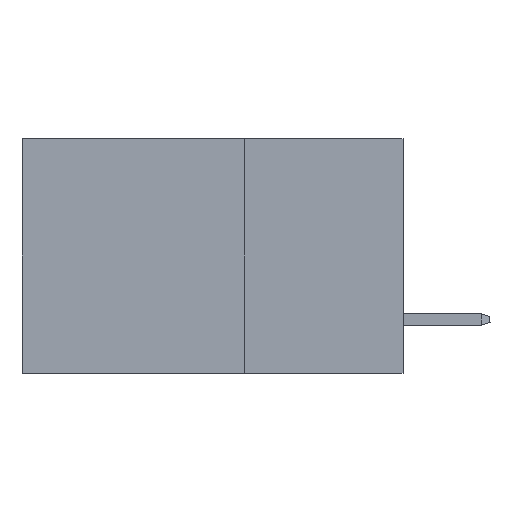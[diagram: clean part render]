
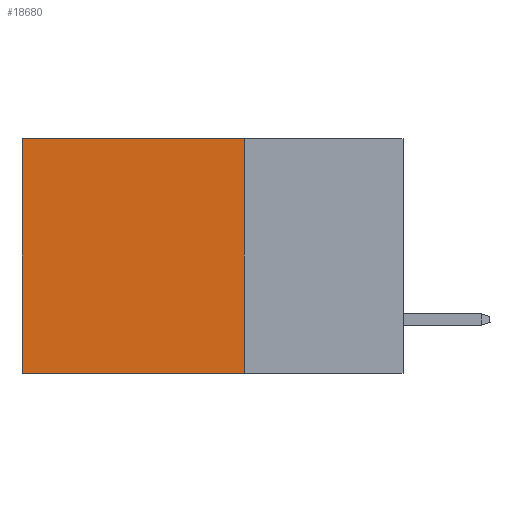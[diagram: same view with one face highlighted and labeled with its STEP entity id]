
A CAD part, left-side view. The second image highlights one B-rep face of the part: STEP entity #18680.
In plain terms, the highlighted planar face has unit normal (-1, 0, 0).
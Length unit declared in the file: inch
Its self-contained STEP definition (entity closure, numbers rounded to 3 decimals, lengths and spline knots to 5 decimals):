
#714 = VERTEX_POINT ( 'NONE', #31569 ) ;
#749 = EDGE_CURVE ( 'NONE', #714, #7709, #8805, .T. ) ;
#1723 = CARTESIAN_POINT ( 'NONE',  ( 0.2875, 0.25, -0.37 ) ) ;
#1878 = VECTOR ( 'NONE', #32065, 39.37008 ) ;
#2256 = EDGE_CURVE ( 'NONE', #714, #27507, #20958, .T. ) ;
#2496 = ORIENTED_EDGE ( 'NONE', *, *, #749, .T. ) ;
#4254 = CARTESIAN_POINT ( 'NONE',  ( 0.2875, 0.6, 0. ) ) ;
#4270 = AXIS2_PLACEMENT_3D ( 'NONE', #32503, #4334, #15008 ) ;
#4334 = DIRECTION ( 'NONE',  ( 1., 0., 0. ) ) ;
#6337 = CARTESIAN_POINT ( 'NONE',  ( 0.2875, 0.6, -0.37 ) ) ;
#7709 = VERTEX_POINT ( 'NONE', #4254 ) ;
#8805 = LINE ( 'NONE', #17120, #1878 ) ;
#9119 = VECTOR ( 'NONE', #20047, 39.37008 ) ;
#9361 = CARTESIAN_POINT ( 'NONE',  ( 0.2875, 0.6, 0. ) ) ;
#11059 = VERTEX_POINT ( 'NONE', #6337 ) ;
#12027 = CARTESIAN_POINT ( 'NONE',  ( 0.2875, 0.25, -0.37 ) ) ;
#14786 = LINE ( 'NONE', #1723, #25663 ) ;
#14794 = LINE ( 'NONE', #9361, #9119 ) ;
#15008 = DIRECTION ( 'NONE',  ( 0., 0., -1. ) ) ;
#16654 = ORIENTED_EDGE ( 'NONE', *, *, #2256, .F. ) ;
#17120 = CARTESIAN_POINT ( 'NONE',  ( 0.2875, 0.25, 0. ) ) ;
#17383 = PLANE ( 'NONE',  #4270 ) ;
#18680 = ADVANCED_FACE ( 'NONE', ( #29951 ), #17383, .F. ) ;
#20047 = DIRECTION ( 'NONE',  ( 0., 0., -1. ) ) ;
#20958 = LINE ( 'NONE', #26386, #22323 ) ;
#21044 = ORIENTED_EDGE ( 'NONE', *, *, #30839, .F. ) ;
#22323 = VECTOR ( 'NONE', #31306, 39.37008 ) ;
#23181 = EDGE_LOOP ( 'NONE', ( #26170, #21044, #16654, #2496 ) ) ;
#25106 = EDGE_CURVE ( 'NONE', #7709, #11059, #14794, .T. ) ;
#25663 = VECTOR ( 'NONE', #29731, 39.37008 ) ;
#26170 = ORIENTED_EDGE ( 'NONE', *, *, #25106, .T. ) ;
#26386 = CARTESIAN_POINT ( 'NONE',  ( 0.2875, 0.25, 0. ) ) ;
#27507 = VERTEX_POINT ( 'NONE', #12027 ) ;
#29731 = DIRECTION ( 'NONE',  ( 0., 1., 0. ) ) ;
#29951 = FACE_OUTER_BOUND ( 'NONE', #23181, .T. ) ;
#30839 = EDGE_CURVE ( 'NONE', #27507, #11059, #14786, .T. ) ;
#31306 = DIRECTION ( 'NONE',  ( 0., 0., -1. ) ) ;
#31569 = CARTESIAN_POINT ( 'NONE',  ( 0.2875, 0.25, 0. ) ) ;
#32065 = DIRECTION ( 'NONE',  ( 0., 1., 0. ) ) ;
#32503 = CARTESIAN_POINT ( 'NONE',  ( 0.2875, 0.25, 0. ) ) ;
